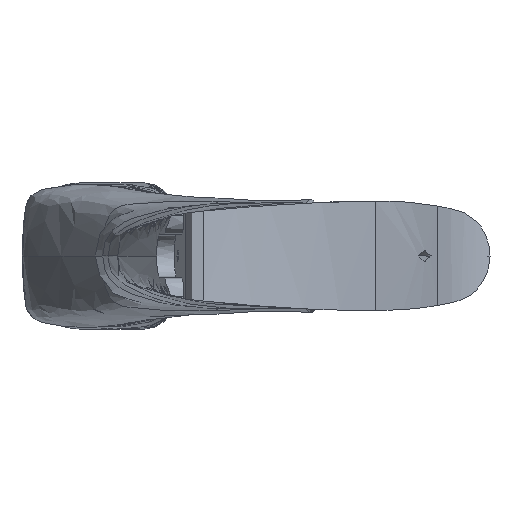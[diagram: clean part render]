
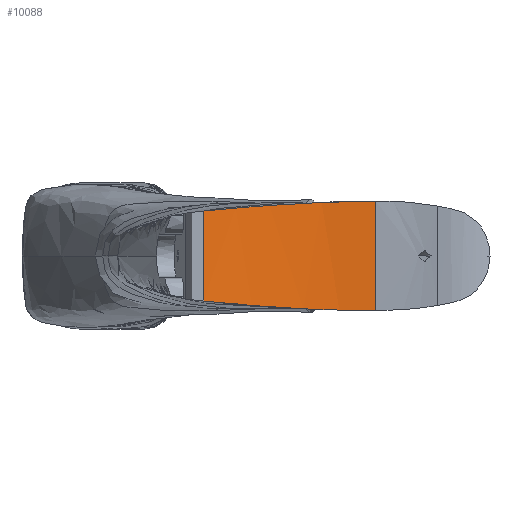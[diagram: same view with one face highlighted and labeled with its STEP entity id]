
A CAD part, left-side view. The second image highlights one B-rep face of the part: STEP entity #10088.
In plain terms, the highlighted cylindrical face has radius 110 mm (diameter 220 mm), a partial arc.
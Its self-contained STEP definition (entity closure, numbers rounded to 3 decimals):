
#217 = CARTESIAN_POINT ( 'NONE',  ( -302.571, -84.144, -17.661 ) ) ;
#288 = B_SPLINE_CURVE_WITH_KNOTS ( 'NONE', 3,
 ( #4684, #11489, #4493, #1514, #496, #7476, #7570, #217, #14464, #10187, #15956, #6172, #8606, #11764 ),
 .UNSPECIFIED., .F., .F.,
 ( 4, 2, 2, 2, 2, 2, 4 ),
 ( -0.061, -0.046, -0.03, -0.027, -0.023, -0.015, 0. ),
 .UNSPECIFIED. ) ;
#339 = CARTESIAN_POINT ( 'NONE',  ( -299.657, -104.214, 18.365 ) ) ;
#436 = LINE ( 'NONE', #6111, #6765 ) ;
#496 = CARTESIAN_POINT ( 'NONE',  ( -305.234, -74.382, -17.096 ) ) ;
#620 = CARTESIAN_POINT ( 'NONE',  ( -308.391, -66.356, 16.374 ) ) ;
#973 = FACE_OUTER_BOUND ( 'NONE', #5101, .T. ) ;
#1431 = CARTESIAN_POINT ( 'NONE',  ( -315.976, -51.677, -27.536 ) ) ;
#1514 = CARTESIAN_POINT ( 'NONE',  ( -306.938, -69.658, -16.736 ) ) ;
#1735 = CARTESIAN_POINT ( 'NONE',  ( -301.394, -89.22, 17.882 ) ) ;
#3314 = CARTESIAN_POINT ( 'NONE',  ( -304.466, -77.061, 17.179 ) ) ;
#3407 = CARTESIAN_POINT ( 'NONE',  ( -305.233, -74.661, 17.014 ) ) ;
#4473 = CARTESIAN_POINT ( 'NONE',  ( -315.976, -51.677, 15.06 ) ) ;
#4493 = CARTESIAN_POINT ( 'NONE',  ( -310.976, -60.47, -15.942 ) ) ;
#4684 = CARTESIAN_POINT ( 'NONE',  ( -315.976, -51.677, -15.084 ) ) ;
#4702 = ORIENTED_EDGE ( 'NONE', *, *, #13958, .T. ) ;
#4809 = CARTESIAN_POINT ( 'NONE',  ( -300.012, -99.17, 18.247 ) ) ;
#5101 = EDGE_LOOP ( 'NONE', ( #11711, #5796, #4702, #5341 ) ) ;
#5341 = ORIENTED_EDGE ( 'NONE', *, *, #16701, .F. ) ;
#5796 = ORIENTED_EDGE ( 'NONE', *, *, #16071, .T. ) ;
#6111 = CARTESIAN_POINT ( 'NONE',  ( -299.657, -109.331, -27.536 ) ) ;
#6172 = CARTESIAN_POINT ( 'NONE',  ( -300.01, -99.163, -18.197 ) ) ;
#6205 = DIRECTION ( 'NONE',  ( 0., 0., 1. ) ) ;
#6387 = VERTEX_POINT ( 'NONE', #9504 ) ;
#6475 = DIRECTION ( 'NONE',  ( 0., 0., 1. ) ) ;
#6765 = VECTOR ( 'NONE', #6205, 1000. ) ;
#7119 = DIRECTION ( 'NONE',  ( 0., 0., 1. ) ) ;
#7476 = CARTESIAN_POINT ( 'NONE',  ( -303.506, -80.456, -17.462 ) ) ;
#7570 = CARTESIAN_POINT ( 'NONE',  ( -303.181, -81.68, -17.532 ) ) ;
#7792 = CARTESIAN_POINT ( 'NONE',  ( -306.959, -69.899, 16.658 ) ) ;
#7865 = AXIS2_PLACEMENT_3D ( 'NONE', #13736, #6475, #11969 ) ;
#8518 = B_SPLINE_CURVE_WITH_KNOTS ( 'NONE', 3,
 ( #14496, #339, #4809, #1735, #16179, #3314, #3407, #14785, #7792, #13377, #620, #14591, #11982, #15893 ),
 .UNSPECIFIED., .F., .F.,
 ( 4, 2, 2, 2, 2, 2, 4 ),
 ( 0.021, 0.036, 0.051, 0.059, 0.063, 0.067, 0.082 ),
 .UNSPECIFIED. ) ;
#8606 = CARTESIAN_POINT ( 'NONE',  ( -299.657, -104.227, -18.266 ) ) ;
#9081 = CARTESIAN_POINT ( 'NONE',  ( -299.657, -109.331, -18.278 ) ) ;
#9370 = CYLINDRICAL_SURFACE ( 'NONE', #7865, 110. ) ;
#9504 = CARTESIAN_POINT ( 'NONE',  ( -299.657, -109.331, 18.42 ) ) ;
#10088 = ADVANCED_FACE ( 'NONE', ( #973 ), #9370, .F. ) ;
#10187 = CARTESIAN_POINT ( 'NONE',  ( -301.498, -89.125, -17.888 ) ) ;
#11489 = CARTESIAN_POINT ( 'NONE',  ( -313.311, -56.007, -15.509 ) ) ;
#11671 = EDGE_CURVE ( 'NONE', #15973, #14292, #288, .T. ) ;
#11711 = ORIENTED_EDGE ( 'NONE', *, *, #11671, .T. ) ;
#11764 = CARTESIAN_POINT ( 'NONE',  ( -299.657, -109.331, -18.278 ) ) ;
#11969 = DIRECTION ( 'NONE',  ( 1., 0., 0. ) ) ;
#11982 = CARTESIAN_POINT ( 'NONE',  ( -313.303, -56.02, 15.469 ) ) ;
#12829 = VERTEX_POINT ( 'NONE', #4473 ) ;
#13377 = CARTESIAN_POINT ( 'NONE',  ( -307.899, -67.534, 16.47 ) ) ;
#13736 = CARTESIAN_POINT ( 'NONE',  ( -409.657, -109.331, -27.536 ) ) ;
#13958 = EDGE_CURVE ( 'NONE', #6387, #12829, #8518, .T. ) ;
#14292 = VERTEX_POINT ( 'NONE', #9081 ) ;
#14464 = CARTESIAN_POINT ( 'NONE',  ( -302.287, -85.387, -17.721 ) ) ;
#14496 = CARTESIAN_POINT ( 'NONE',  ( -299.657, -109.331, 18.42 ) ) ;
#14591 = CARTESIAN_POINT ( 'NONE',  ( -310.946, -60.524, 15.886 ) ) ;
#14785 = CARTESIAN_POINT ( 'NONE',  ( -306.511, -71.086, 16.749 ) ) ;
#15438 = CARTESIAN_POINT ( 'NONE',  ( -315.976, -51.677, -15.084 ) ) ;
#15893 = CARTESIAN_POINT ( 'NONE',  ( -315.976, -51.677, 15.06 ) ) ;
#15956 = CARTESIAN_POINT ( 'NONE',  ( -301.061, -91.627, -17.979 ) ) ;
#15973 = VERTEX_POINT ( 'NONE', #15438 ) ;
#16071 = EDGE_CURVE ( 'NONE', #14292, #6387, #436, .T. ) ;
#16179 = CARTESIAN_POINT ( 'NONE',  ( -302.421, -84.315, 17.634 ) ) ;
#16701 = EDGE_CURVE ( 'NONE', #15973, #12829, #17093, .T. ) ;
#17093 = LINE ( 'NONE', #1431, #18322 ) ;
#18322 = VECTOR ( 'NONE', #7119, 1000. ) ;
